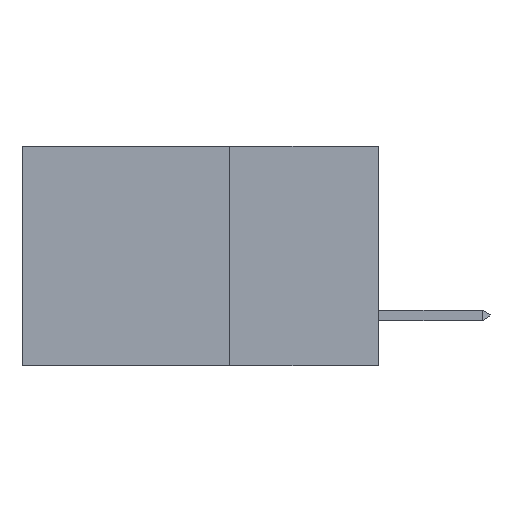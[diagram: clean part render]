
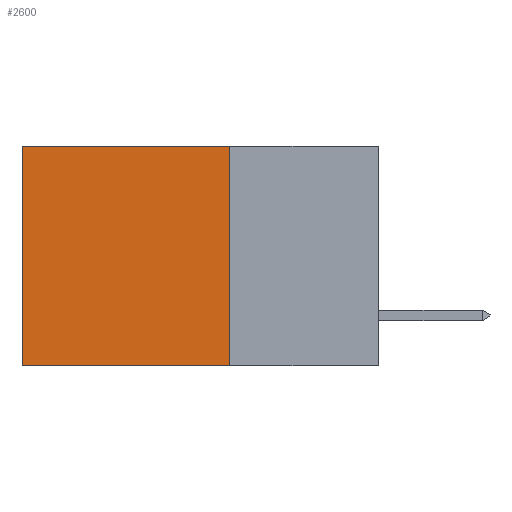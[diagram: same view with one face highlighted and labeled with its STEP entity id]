
A CAD part, left-side view. The second image highlights one B-rep face of the part: STEP entity #2600.
In plain terms, the highlighted planar face has unit normal (-1, 0, 0).
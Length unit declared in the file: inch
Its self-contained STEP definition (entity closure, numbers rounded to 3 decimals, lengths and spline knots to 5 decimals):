
#210 = EDGE_CURVE ( 'NONE', #4137, #8371, #4326, .T. ) ;
#345 = EDGE_CURVE ( 'NONE', #2164, #9056, #961, .T. ) ;
#796 = FACE_OUTER_BOUND ( 'NONE', #1264, .T. ) ;
#800 = ORIENTED_EDGE ( 'NONE', *, *, #2469, .T. ) ;
#961 = LINE ( 'NONE', #6144, #7076 ) ;
#1264 = EDGE_LOOP ( 'NONE', ( #800, #5528, #6211, #8786 ) ) ;
#1675 = CARTESIAN_POINT ( 'NONE',  ( 0.298, 0.25, -0.37 ) ) ;
#1734 = CARTESIAN_POINT ( 'NONE',  ( 0.298, 0.25, 0. ) ) ;
#2164 = VERTEX_POINT ( 'NONE', #1734 ) ;
#2287 = VECTOR ( 'NONE', #9887, 39.37008 ) ;
#2469 = EDGE_CURVE ( 'NONE', #9056, #8371, #8203, .T. ) ;
#2600 = ADVANCED_FACE ( 'NONE', ( #796 ), #6029, .F. ) ;
#3032 = LINE ( 'NONE', #8257, #2287 ) ;
#3313 = DIRECTION ( 'NONE',  ( 0., 0., -1. ) ) ;
#3848 = VECTOR ( 'NONE', #9684, 39.37008 ) ;
#3953 = CARTESIAN_POINT ( 'NONE',  ( 0.298, 0.6, 0. ) ) ;
#4137 = VERTEX_POINT ( 'NONE', #6187 ) ;
#4324 = DIRECTION ( 'NONE',  ( 0., 0., -1. ) ) ;
#4326 = LINE ( 'NONE', #1675, #3848 ) ;
#4363 = CARTESIAN_POINT ( 'NONE',  ( 0.298, 0.6, 0. ) ) ;
#4675 = AXIS2_PLACEMENT_3D ( 'NONE', #9299, #8110, #3313 ) ;
#5165 = EDGE_CURVE ( 'NONE', #2164, #4137, #3032, .T. ) ;
#5528 = ORIENTED_EDGE ( 'NONE', *, *, #210, .F. ) ;
#6029 = PLANE ( 'NONE',  #4675 ) ;
#6144 = CARTESIAN_POINT ( 'NONE',  ( 0.298, 0.25, 0. ) ) ;
#6187 = CARTESIAN_POINT ( 'NONE',  ( 0.298, 0.25, -0.37 ) ) ;
#6211 = ORIENTED_EDGE ( 'NONE', *, *, #5165, .F. ) ;
#7076 = VECTOR ( 'NONE', #9337, 39.37008 ) ;
#7700 = CARTESIAN_POINT ( 'NONE',  ( 0.298, 0.6, -0.37 ) ) ;
#8110 = DIRECTION ( 'NONE',  ( 1., 0., 0. ) ) ;
#8203 = LINE ( 'NONE', #4363, #8321 ) ;
#8257 = CARTESIAN_POINT ( 'NONE',  ( 0.298, 0.25, 0. ) ) ;
#8321 = VECTOR ( 'NONE', #4324, 39.37008 ) ;
#8371 = VERTEX_POINT ( 'NONE', #7700 ) ;
#8786 = ORIENTED_EDGE ( 'NONE', *, *, #345, .T. ) ;
#9056 = VERTEX_POINT ( 'NONE', #3953 ) ;
#9299 = CARTESIAN_POINT ( 'NONE',  ( 0.298, 0.25, 0. ) ) ;
#9337 = DIRECTION ( 'NONE',  ( 0., 1., 0. ) ) ;
#9684 = DIRECTION ( 'NONE',  ( 0., 1., 0. ) ) ;
#9887 = DIRECTION ( 'NONE',  ( 0., 0., -1. ) ) ;
